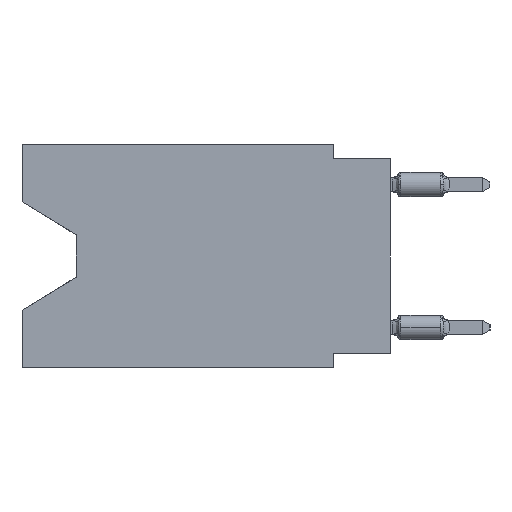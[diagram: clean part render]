
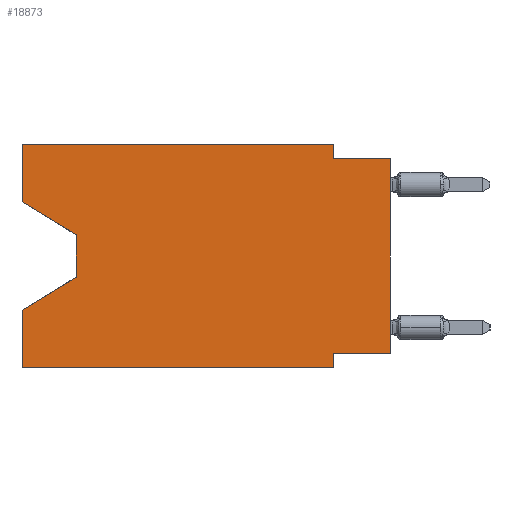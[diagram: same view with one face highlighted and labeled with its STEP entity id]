
A CAD part, left-side view. The second image highlights one B-rep face of the part: STEP entity #18873.
In plain terms, the highlighted planar face has unit normal (-1, 0, 0).
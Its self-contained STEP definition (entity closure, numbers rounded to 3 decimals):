
#573 = VERTEX_POINT ( 'NONE', #22325 ) ;
#735 = CARTESIAN_POINT ( 'NONE',  ( 0., 2.54, -9.271 ) ) ;
#1046 = VECTOR ( 'NONE', #5896, 1000. ) ;
#1363 = CARTESIAN_POINT ( 'NONE',  ( 0., 0., -0.635 ) ) ;
#1635 = PLANE ( 'NONE',  #8603 ) ;
#1732 = ORIENTED_EDGE ( 'NONE', *, *, #9481, .T. ) ;
#1745 = CARTESIAN_POINT ( 'NONE',  ( 0., 2.54, -9.906 ) ) ;
#2183 = VERTEX_POINT ( 'NONE', #4201 ) ;
#2898 = ORIENTED_EDGE ( 'NONE', *, *, #10077, .F. ) ;
#3076 = LINE ( 'NONE', #12914, #8893 ) ;
#3077 = LINE ( 'NONE', #12438, #19069 ) ;
#3285 = VECTOR ( 'NONE', #18790, 1000. ) ;
#3674 = CARTESIAN_POINT ( 'NONE',  ( 0., 0., -9.271 ) ) ;
#4201 = CARTESIAN_POINT ( 'NONE',  ( 0., 16.383, -2.546 ) ) ;
#4292 = VERTEX_POINT ( 'NONE', #22269 ) ;
#4406 = VECTOR ( 'NONE', #14933, 1000. ) ;
#4460 = EDGE_CURVE ( 'NONE', #19067, #13229, #3076, .T. ) ;
#4664 = CARTESIAN_POINT ( 'NONE',  ( 0., 16.383, 0. ) ) ;
#4922 = EDGE_CURVE ( 'NONE', #4292, #573, #25162, .T. ) ;
#5069 = CARTESIAN_POINT ( 'NONE',  ( 0., 0., -9.271 ) ) ;
#5628 = CARTESIAN_POINT ( 'NONE',  ( 0., 16.383, -7.36 ) ) ;
#5755 = EDGE_CURVE ( 'NONE', #24150, #13210, #14549, .T. ) ;
#5896 = DIRECTION ( 'NONE',  ( 0., 0., -1. ) ) ;
#6020 = DIRECTION ( 'NONE',  ( 0., 0., 1. ) ) ;
#6045 = VECTOR ( 'NONE', #9811, 1000. ) ;
#6576 = ORIENTED_EDGE ( 'NONE', *, *, #16032, .T. ) ;
#6639 = LINE ( 'NONE', #5069, #3285 ) ;
#7041 = LINE ( 'NONE', #10940, #4406 ) ;
#7841 = LINE ( 'NONE', #23242, #1046 ) ;
#8570 = EDGE_CURVE ( 'NONE', #2183, #4292, #14295, .T. ) ;
#8603 = AXIS2_PLACEMENT_3D ( 'NONE', #21164, #17138, #19234 ) ;
#8701 = EDGE_CURVE ( 'NONE', #19207, #18776, #6639, .T. ) ;
#8893 = VECTOR ( 'NONE', #15238, 1000. ) ;
#8903 = LINE ( 'NONE', #16780, #19695 ) ;
#8984 = CARTESIAN_POINT ( 'NONE',  ( 0., 16.383, -9.906 ) ) ;
#9404 = CARTESIAN_POINT ( 'NONE',  ( 0., 2.54, -9.906 ) ) ;
#9481 = EDGE_CURVE ( 'NONE', #22471, #25291, #3077, .T. ) ;
#9482 = CARTESIAN_POINT ( 'NONE',  ( 0., 16.383, 0. ) ) ;
#9811 = DIRECTION ( 'NONE',  ( 0., 0., -1. ) ) ;
#10077 = EDGE_CURVE ( 'NONE', #24150, #25291, #22395, .T. ) ;
#10485 = VECTOR ( 'NONE', #11611, 1000. ) ;
#10940 = CARTESIAN_POINT ( 'NONE',  ( 0., 0., 0. ) ) ;
#11183 = CARTESIAN_POINT ( 'NONE',  ( 0., 16.383, -9.906 ) ) ;
#11611 = DIRECTION ( 'NONE',  ( 0., 0., -1. ) ) ;
#12438 = CARTESIAN_POINT ( 'NONE',  ( 0., 13.97, -5.893 ) ) ;
#12571 = DIRECTION ( 'NONE',  ( 0., 0., 1. ) ) ;
#12914 = CARTESIAN_POINT ( 'NONE',  ( 0., 0., -0.635 ) ) ;
#13210 = VERTEX_POINT ( 'NONE', #9404 ) ;
#13229 = VERTEX_POINT ( 'NONE', #1363 ) ;
#14032 = CARTESIAN_POINT ( 'NONE',  ( 0., 13.97, -5.893 ) ) ;
#14295 = LINE ( 'NONE', #22201, #22710 ) ;
#14549 = LINE ( 'NONE', #8984, #16389 ) ;
#14840 = DIRECTION ( 'NONE',  ( 0., -0.855, -0.519 ) ) ;
#14923 = DIRECTION ( 'NONE',  ( 0., -1., 0. ) ) ;
#14933 = DIRECTION ( 'NONE',  ( 0., 0., 1. ) ) ;
#15238 = DIRECTION ( 'NONE',  ( 0., -1., 0. ) ) ;
#15354 = VECTOR ( 'NONE', #12571, 1000. ) ;
#15595 = ORIENTED_EDGE ( 'NONE', *, *, #20143, .T. ) ;
#15678 = CARTESIAN_POINT ( 'NONE',  ( 0., 13.97, -4.013 ) ) ;
#16032 = EDGE_CURVE ( 'NONE', #2183, #22829, #8903, .T. ) ;
#16062 = EDGE_CURVE ( 'NONE', #573, #19067, #23539, .T. ) ;
#16389 = VECTOR ( 'NONE', #14923, 1000. ) ;
#16494 = ORIENTED_EDGE ( 'NONE', *, *, #16062, .F. ) ;
#16780 = CARTESIAN_POINT ( 'NONE',  ( 0., 16.383, -2.546 ) ) ;
#16838 = ORIENTED_EDGE ( 'NONE', *, *, #4460, .F. ) ;
#17138 = DIRECTION ( 'NONE',  ( 1., 0., 0. ) ) ;
#17168 = CARTESIAN_POINT ( 'NONE',  ( 0., 2.54, 0. ) ) ;
#17361 = DIRECTION ( 'NONE',  ( 0., -1., 0. ) ) ;
#18776 = VERTEX_POINT ( 'NONE', #735 ) ;
#18790 = DIRECTION ( 'NONE',  ( 0., 1., 0. ) ) ;
#18873 = ADVANCED_FACE ( 'NONE', ( #25461 ), #1635, .F. ) ;
#19002 = ORIENTED_EDGE ( 'NONE', *, *, #5755, .T. ) ;
#19067 = VERTEX_POINT ( 'NONE', #24771 ) ;
#19069 = VECTOR ( 'NONE', #20690, 1000. ) ;
#19207 = VERTEX_POINT ( 'NONE', #3674 ) ;
#19234 = DIRECTION ( 'NONE',  ( 0., 0., -1. ) ) ;
#19695 = VECTOR ( 'NONE', #14840, 1000. ) ;
#19936 = EDGE_LOOP ( 'NONE', ( #6576, #15595, #1732, #2898, #19002, #22136, #20556, #20212, #16838, #16494, #22585, #23042 ) ) ;
#20143 = EDGE_CURVE ( 'NONE', #22829, #22471, #7841, .T. ) ;
#20212 = ORIENTED_EDGE ( 'NONE', *, *, #21446, .T. ) ;
#20493 = VECTOR ( 'NONE', #17361, 1000. ) ;
#20556 = ORIENTED_EDGE ( 'NONE', *, *, #8701, .F. ) ;
#20690 = DIRECTION ( 'NONE',  ( 0., 0.855, -0.519 ) ) ;
#21164 = CARTESIAN_POINT ( 'NONE',  ( 0., 16.383, 0. ) ) ;
#21446 = EDGE_CURVE ( 'NONE', #19207, #13229, #7041, .T. ) ;
#21549 = LINE ( 'NONE', #1745, #10485 ) ;
#22136 = ORIENTED_EDGE ( 'NONE', *, *, #25237, .F. ) ;
#22201 = CARTESIAN_POINT ( 'NONE',  ( 0., 16.383, 0. ) ) ;
#22269 = CARTESIAN_POINT ( 'NONE',  ( 0., 16.383, 0. ) ) ;
#22325 = CARTESIAN_POINT ( 'NONE',  ( 0., 2.54, 0. ) ) ;
#22395 = LINE ( 'NONE', #4664, #15354 ) ;
#22471 = VERTEX_POINT ( 'NONE', #14032 ) ;
#22585 = ORIENTED_EDGE ( 'NONE', *, *, #4922, .F. ) ;
#22710 = VECTOR ( 'NONE', #6020, 1000. ) ;
#22829 = VERTEX_POINT ( 'NONE', #15678 ) ;
#23042 = ORIENTED_EDGE ( 'NONE', *, *, #8570, .F. ) ;
#23242 = CARTESIAN_POINT ( 'NONE',  ( 0., 13.97, -4.013 ) ) ;
#23539 = LINE ( 'NONE', #17168, #6045 ) ;
#24150 = VERTEX_POINT ( 'NONE', #11183 ) ;
#24771 = CARTESIAN_POINT ( 'NONE',  ( 0., 2.54, -0.635 ) ) ;
#25162 = LINE ( 'NONE', #9482, #20493 ) ;
#25237 = EDGE_CURVE ( 'NONE', #18776, #13210, #21549, .T. ) ;
#25291 = VERTEX_POINT ( 'NONE', #5628 ) ;
#25461 = FACE_OUTER_BOUND ( 'NONE', #19936, .T. ) ;
